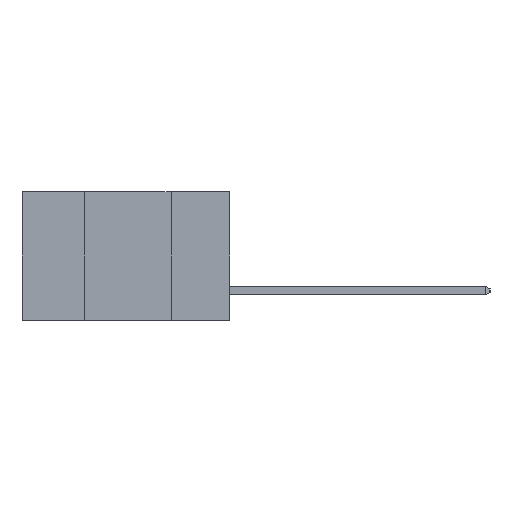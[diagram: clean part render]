
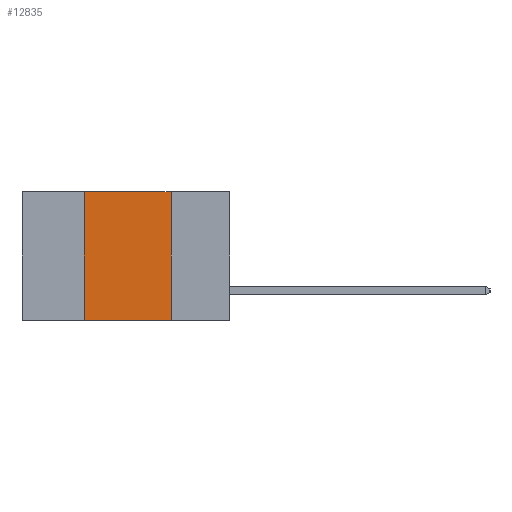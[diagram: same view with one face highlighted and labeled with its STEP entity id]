
A CAD part, left-side view. The second image highlights one B-rep face of the part: STEP entity #12835.
In plain terms, the highlighted planar face has unit normal (-1, 0, 0).
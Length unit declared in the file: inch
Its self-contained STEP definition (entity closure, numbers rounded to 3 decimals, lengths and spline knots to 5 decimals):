
#41 = FACE_OUTER_BOUND ( 'NONE', #5347, .T. ) ;
#669 = DIRECTION ( 'NONE',  ( 1., 0., 0. ) ) ;
#1329 = CARTESIAN_POINT ( 'NONE',  ( 0., 0.17, 0. ) ) ;
#2042 = LINE ( 'NONE', #12018, #12543 ) ;
#2805 = AXIS2_PLACEMENT_3D ( 'NONE', #6802, #669, #7851 ) ;
#3380 = DIRECTION ( 'NONE',  ( 0., 0., 1. ) ) ;
#3724 = PLANE ( 'NONE',  #2805 ) ;
#4426 = EDGE_CURVE ( 'NONE', #8586, #7595, #10040, .T. ) ;
#4779 = VERTEX_POINT ( 'NONE', #7057 ) ;
#5347 = EDGE_LOOP ( 'NONE', ( #6337, #6672, #6443, #6513 ) ) ;
#5421 = EDGE_CURVE ( 'NONE', #7595, #5478, #12045, .T. ) ;
#5478 = VERTEX_POINT ( 'NONE', #1329 ) ;
#5512 = EDGE_CURVE ( 'NONE', #5478, #4779, #8285, .T. ) ;
#6337 = ORIENTED_EDGE ( 'NONE', *, *, #5512, .F. ) ;
#6443 = ORIENTED_EDGE ( 'NONE', *, *, #4426, .F. ) ;
#6513 = ORIENTED_EDGE ( 'NONE', *, *, #8318, .T. ) ;
#6672 = ORIENTED_EDGE ( 'NONE', *, *, #5421, .F. ) ;
#6802 = CARTESIAN_POINT ( 'NONE',  ( 0., 0.6, 0. ) ) ;
#7057 = CARTESIAN_POINT ( 'NONE',  ( 0., 0.17, -0.37 ) ) ;
#7340 = VECTOR ( 'NONE', #3380, 39.37008 ) ;
#7475 = DIRECTION ( 'NONE',  ( 0., -1., 0. ) ) ;
#7595 = VERTEX_POINT ( 'NONE', #9051 ) ;
#7851 = DIRECTION ( 'NONE',  ( 0., 0., -1. ) ) ;
#8285 = LINE ( 'NONE', #11902, #10615 ) ;
#8318 = EDGE_CURVE ( 'NONE', #8586, #4779, #2042, .T. ) ;
#8586 = VERTEX_POINT ( 'NONE', #9076 ) ;
#9051 = CARTESIAN_POINT ( 'NONE',  ( 0., 0.42, 0. ) ) ;
#9076 = CARTESIAN_POINT ( 'NONE',  ( 0., 0.42, -0.37 ) ) ;
#9194 = CARTESIAN_POINT ( 'NONE',  ( 0., 0.6, 0. ) ) ;
#10040 = LINE ( 'NONE', #12476, #7340 ) ;
#10193 = DIRECTION ( 'NONE',  ( 0., -1., 0. ) ) ;
#10615 = VECTOR ( 'NONE', #12580, 39.37008 ) ;
#11765 = VECTOR ( 'NONE', #7475, 39.37008 ) ;
#11902 = CARTESIAN_POINT ( 'NONE',  ( 0., 0.17, 0. ) ) ;
#12018 = CARTESIAN_POINT ( 'NONE',  ( 0., 0.6, -0.37 ) ) ;
#12045 = LINE ( 'NONE', #9194, #11765 ) ;
#12476 = CARTESIAN_POINT ( 'NONE',  ( 0., 0.42, 0. ) ) ;
#12543 = VECTOR ( 'NONE', #10193, 39.37008 ) ;
#12580 = DIRECTION ( 'NONE',  ( 0., 0., -1. ) ) ;
#12835 = ADVANCED_FACE ( 'NONE', ( #41 ), #3724, .F. ) ;
